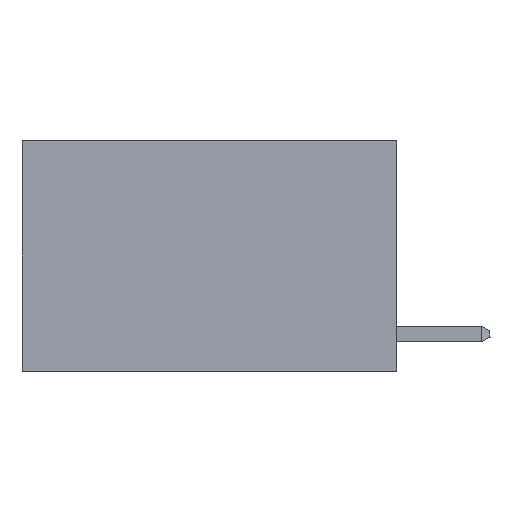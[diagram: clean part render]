
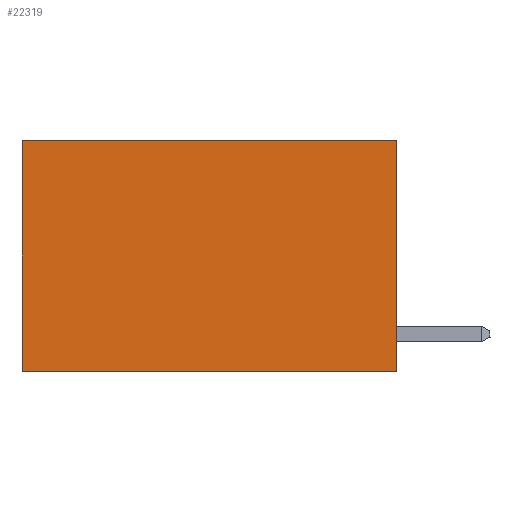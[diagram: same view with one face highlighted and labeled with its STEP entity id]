
A CAD part, left-side view. The second image highlights one B-rep face of the part: STEP entity #22319.
In plain terms, the highlighted planar face has unit normal (-1, 0, 0).
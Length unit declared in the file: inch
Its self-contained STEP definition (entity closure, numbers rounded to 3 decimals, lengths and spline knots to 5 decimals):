
#127 = CARTESIAN_POINT ( 'NONE',  ( 0.2625, 0., -0.37 ) ) ;
#601 = CARTESIAN_POINT ( 'NONE',  ( 0.2625, 0., 0. ) ) ;
#938 = VERTEX_POINT ( 'NONE', #127 ) ;
#1002 = EDGE_CURVE ( 'NONE', #938, #16116, #10756, .T. ) ;
#1167 = LINE ( 'NONE', #1284, #15041 ) ;
#1284 = CARTESIAN_POINT ( 'NONE',  ( 0.2625, 0., 0. ) ) ;
#1415 = LINE ( 'NONE', #4915, #18083 ) ;
#1666 = EDGE_LOOP ( 'NONE', ( #15198, #5997, #14363, #14631 ) ) ;
#2987 = AXIS2_PLACEMENT_3D ( 'NONE', #601, #14067, #21015 ) ;
#4535 = VECTOR ( 'NONE', #16771, 39.37008 ) ;
#4915 = CARTESIAN_POINT ( 'NONE',  ( 0.2625, 0., 0. ) ) ;
#5997 = ORIENTED_EDGE ( 'NONE', *, *, #1002, .F. ) ;
#7262 = VECTOR ( 'NONE', #12898, 39.37008 ) ;
#7328 = VERTEX_POINT ( 'NONE', #18370 ) ;
#8015 = CARTESIAN_POINT ( 'NONE',  ( 0.2625, 0.6, 0. ) ) ;
#8362 = EDGE_CURVE ( 'NONE', #7328, #938, #1167, .T. ) ;
#9055 = VERTEX_POINT ( 'NONE', #11283 ) ;
#10756 = LINE ( 'NONE', #15994, #7262 ) ;
#10778 = EDGE_CURVE ( 'NONE', #9055, #16116, #19942, .T. ) ;
#10820 = CARTESIAN_POINT ( 'NONE',  ( 0.2625, 0.6, -0.37 ) ) ;
#11283 = CARTESIAN_POINT ( 'NONE',  ( 0.2625, 0.6, 0. ) ) ;
#12898 = DIRECTION ( 'NONE',  ( 0., 1., 0. ) ) ;
#13743 = DIRECTION ( 'NONE',  ( 0., 1., 0. ) ) ;
#14067 = DIRECTION ( 'NONE',  ( 1., 0., 0. ) ) ;
#14363 = ORIENTED_EDGE ( 'NONE', *, *, #8362, .F. ) ;
#14631 = ORIENTED_EDGE ( 'NONE', *, *, #15142, .T. ) ;
#15000 = DIRECTION ( 'NONE',  ( 0., 0., -1. ) ) ;
#15041 = VECTOR ( 'NONE', #15000, 39.37008 ) ;
#15142 = EDGE_CURVE ( 'NONE', #7328, #9055, #1415, .T. ) ;
#15198 = ORIENTED_EDGE ( 'NONE', *, *, #10778, .T. ) ;
#15994 = CARTESIAN_POINT ( 'NONE',  ( 0.2625, 0., -0.37 ) ) ;
#16116 = VERTEX_POINT ( 'NONE', #10820 ) ;
#16244 = FACE_OUTER_BOUND ( 'NONE', #1666, .T. ) ;
#16771 = DIRECTION ( 'NONE',  ( 0., 0., -1. ) ) ;
#18083 = VECTOR ( 'NONE', #13743, 39.37008 ) ;
#18370 = CARTESIAN_POINT ( 'NONE',  ( 0.2625, 0., 0. ) ) ;
#19194 = PLANE ( 'NONE',  #2987 ) ;
#19942 = LINE ( 'NONE', #8015, #4535 ) ;
#21015 = DIRECTION ( 'NONE',  ( 0., 0., -1. ) ) ;
#22319 = ADVANCED_FACE ( 'NONE', ( #16244 ), #19194, .F. ) ;
